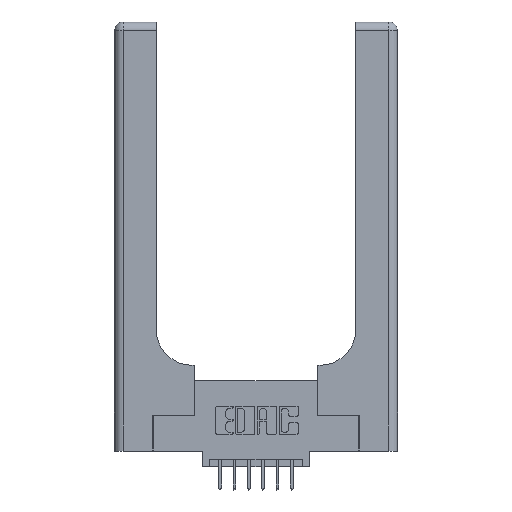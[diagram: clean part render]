
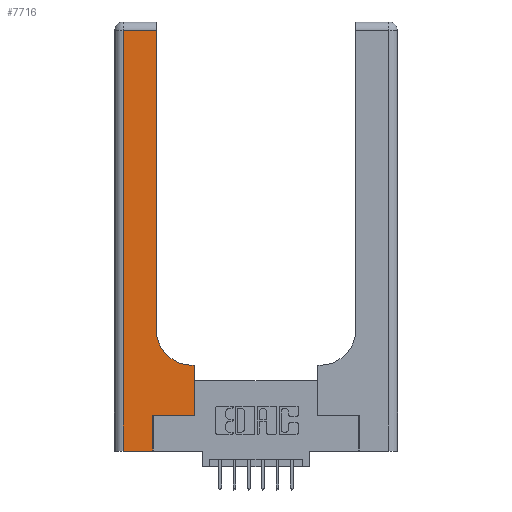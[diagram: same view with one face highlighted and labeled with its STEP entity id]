
A CAD part, top view. The second image highlights one B-rep face of the part: STEP entity #7716.
In plain terms, the highlighted planar face has unit normal (0, 0, 1).
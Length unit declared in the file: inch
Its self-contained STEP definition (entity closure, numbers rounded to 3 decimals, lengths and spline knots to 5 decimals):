
#146 = CARTESIAN_POINT ( 'NONE',  ( 0.269, 0., 0.37 ) ) ;
#147 = LINE ( 'NONE', #5925, #10228 ) ;
#405 = LINE ( 'NONE', #9369, #5814 ) ;
#555 = CARTESIAN_POINT ( 'NONE',  ( 0.269, 0., 0.37 ) ) ;
#1359 = DIRECTION ( 'NONE',  ( 0., -1., 0. ) ) ;
#1409 = LINE ( 'NONE', #555, #13701 ) ;
#1584 = DIRECTION ( 'NONE',  ( 1., 0., 0. ) ) ;
#1933 = LINE ( 'NONE', #14269, #11822 ) ;
#1963 = ORIENTED_EDGE ( 'NONE', *, *, #6376, .T. ) ;
#2080 = LINE ( 'NONE', #11217, #13987 ) ;
#2121 = DIRECTION ( 'NONE',  ( 0., 0., -1. ) ) ;
#2155 = EDGE_CURVE ( 'NONE', #8172, #6287, #147, .T. ) ;
#2324 = ORIENTED_EDGE ( 'NONE', *, *, #2155, .T. ) ;
#2419 = VECTOR ( 'NONE', #6432, 39.37008 ) ;
#2476 = CARTESIAN_POINT ( 'NONE',  ( 0., 3., 0.37 ) ) ;
#2923 = CARTESIAN_POINT ( 'NONE',  ( 0.2915, 0.85, 0.37 ) ) ;
#2968 = EDGE_LOOP ( 'NONE', ( #1963, #4315, #2324, #9651, #8406, #9283, #8559, #12358, #5598 ) ) ;
#3674 = VERTEX_POINT ( 'NONE', #13113 ) ;
#3816 = EDGE_CURVE ( 'NONE', #14805, #8172, #12879, .T. ) ;
#3936 = VECTOR ( 'NONE', #9302, 39.37008 ) ;
#4133 = VERTEX_POINT ( 'NONE', #11349 ) ;
#4202 = VECTOR ( 'NONE', #7102, 39.37008 ) ;
#4315 = ORIENTED_EDGE ( 'NONE', *, *, #3816, .T. ) ;
#4338 = DIRECTION ( 'NONE',  ( 0., 1., 0. ) ) ;
#4816 = DIRECTION ( 'NONE',  ( -1., 0., 0. ) ) ;
#5598 = ORIENTED_EDGE ( 'NONE', *, *, #7377, .T. ) ;
#5634 = AXIS2_PLACEMENT_3D ( 'NONE', #2476, #11682, #4816 ) ;
#5814 = VECTOR ( 'NONE', #6045, 39.37008 ) ;
#5925 = CARTESIAN_POINT ( 'NONE',  ( 0.06, 3., 0.37 ) ) ;
#6045 = DIRECTION ( 'NONE',  ( -1., 0., 0. ) ) ;
#6092 = VERTEX_POINT ( 'NONE', #2923 ) ;
#6287 = VERTEX_POINT ( 'NONE', #14940 ) ;
#6376 = EDGE_CURVE ( 'NONE', #6092, #14805, #9414, .T. ) ;
#6400 = CARTESIAN_POINT ( 'NONE',  ( 0.2915, 2.94, 0.37 ) ) ;
#6432 = DIRECTION ( 'NONE',  ( -1., 0., 0. ) ) ;
#6499 = FACE_OUTER_BOUND ( 'NONE', #2968, .T. ) ;
#6596 = EDGE_CURVE ( 'NONE', #8607, #9476, #405, .T. ) ;
#7102 = DIRECTION ( 'NONE',  ( 0., 1., 0. ) ) ;
#7149 = CARTESIAN_POINT ( 'NONE',  ( 0.06, 2.94, 0.37 ) ) ;
#7175 = CARTESIAN_POINT ( 'NONE',  ( 0.5585, 0.6, 0.37 ) ) ;
#7377 = EDGE_CURVE ( 'NONE', #9476, #6092, #12445, .T. ) ;
#7489 = CARTESIAN_POINT ( 'NONE',  ( 0., 2.94, 0.37 ) ) ;
#7580 = AXIS2_PLACEMENT_3D ( 'NONE', #14761, #2121, #7830 ) ;
#7716 = ADVANCED_FACE ( 'NONE', ( #6499 ), #13995, .F. ) ;
#7830 = DIRECTION ( 'NONE',  ( 1., 0., 0. ) ) ;
#8009 = CARTESIAN_POINT ( 'NONE',  ( 0., 0., 0.37 ) ) ;
#8149 = VERTEX_POINT ( 'NONE', #146 ) ;
#8172 = VERTEX_POINT ( 'NONE', #7149 ) ;
#8363 = EDGE_CURVE ( 'NONE', #3674, #4133, #1933, .T. ) ;
#8406 = ORIENTED_EDGE ( 'NONE', *, *, #13983, .T. ) ;
#8559 = ORIENTED_EDGE ( 'NONE', *, *, #9422, .T. ) ;
#8607 = VERTEX_POINT ( 'NONE', #7175 ) ;
#9283 = ORIENTED_EDGE ( 'NONE', *, *, #8363, .T. ) ;
#9302 = DIRECTION ( 'NONE',  ( 1., 0., 0. ) ) ;
#9312 = CARTESIAN_POINT ( 'NONE',  ( 0.2915, 3., 0.37 ) ) ;
#9369 = CARTESIAN_POINT ( 'NONE',  ( 0.2915, 0.6, 0.37 ) ) ;
#9414 = LINE ( 'NONE', #9312, #4202 ) ;
#9422 = EDGE_CURVE ( 'NONE', #4133, #8607, #2080, .T. ) ;
#9476 = VERTEX_POINT ( 'NONE', #10119 ) ;
#9651 = ORIENTED_EDGE ( 'NONE', *, *, #14492, .T. ) ;
#9681 = DIRECTION ( 'NONE',  ( 0., 1., 0. ) ) ;
#10119 = CARTESIAN_POINT ( 'NONE',  ( 0.5415, 0.6, 0.37 ) ) ;
#10228 = VECTOR ( 'NONE', #1359, 39.37008 ) ;
#11217 = CARTESIAN_POINT ( 'NONE',  ( 0.5585, 0.25, 0.37 ) ) ;
#11349 = CARTESIAN_POINT ( 'NONE',  ( 0.5585, 0.25, 0.37 ) ) ;
#11477 = LINE ( 'NONE', #8009, #3936 ) ;
#11682 = DIRECTION ( 'NONE',  ( 0., 0., -1. ) ) ;
#11822 = VECTOR ( 'NONE', #1584, 39.37008 ) ;
#12358 = ORIENTED_EDGE ( 'NONE', *, *, #6596, .T. ) ;
#12445 = CIRCLE ( 'NONE', #7580, 0.25 ) ;
#12879 = LINE ( 'NONE', #7489, #2419 ) ;
#13113 = CARTESIAN_POINT ( 'NONE',  ( 0.269, 0.25, 0.37 ) ) ;
#13701 = VECTOR ( 'NONE', #9681, 39.37008 ) ;
#13983 = EDGE_CURVE ( 'NONE', #8149, #3674, #1409, .T. ) ;
#13987 = VECTOR ( 'NONE', #4338, 39.37008 ) ;
#13995 = PLANE ( 'NONE',  #5634 ) ;
#14269 = CARTESIAN_POINT ( 'NONE',  ( 0.269, 0.25, 0.37 ) ) ;
#14492 = EDGE_CURVE ( 'NONE', #6287, #8149, #11477, .T. ) ;
#14761 = CARTESIAN_POINT ( 'NONE',  ( 0.5415, 0.85, 0.37 ) ) ;
#14805 = VERTEX_POINT ( 'NONE', #6400 ) ;
#14940 = CARTESIAN_POINT ( 'NONE',  ( 0.06, 0., 0.37 ) ) ;
